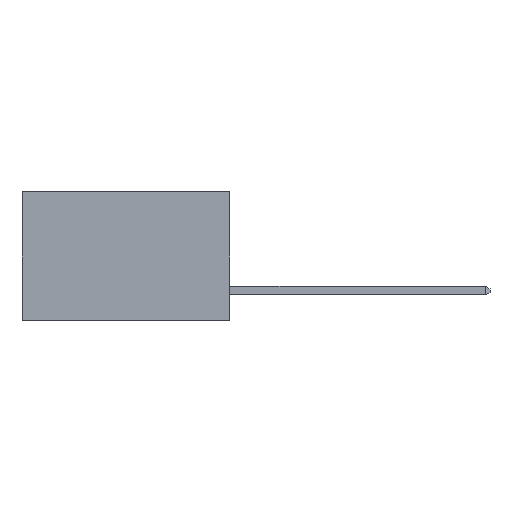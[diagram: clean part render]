
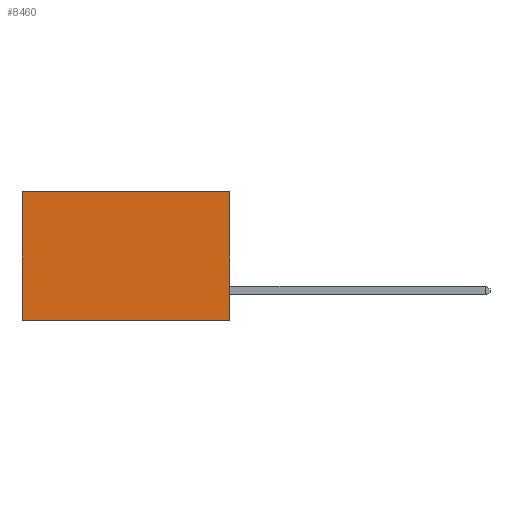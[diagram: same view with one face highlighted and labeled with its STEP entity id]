
A CAD part, left-side view. The second image highlights one B-rep face of the part: STEP entity #8460.
In plain terms, the highlighted planar face has unit normal (-1, 0, 0).
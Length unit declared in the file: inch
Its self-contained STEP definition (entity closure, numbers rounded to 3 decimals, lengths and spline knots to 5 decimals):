
#260 = VECTOR ( 'NONE', #10000, 39.37008 ) ;
#719 = VERTEX_POINT ( 'NONE', #7759 ) ;
#1228 = VERTEX_POINT ( 'NONE', #2418 ) ;
#1392 = CARTESIAN_POINT ( 'NONE',  ( 0.2615, 0., -0.37 ) ) ;
#1958 = LINE ( 'NONE', #9215, #3961 ) ;
#2029 = EDGE_CURVE ( 'NONE', #719, #5924, #1958, .T. ) ;
#2131 = CARTESIAN_POINT ( 'NONE',  ( 0.2615, 0.6, -0.37 ) ) ;
#2418 = CARTESIAN_POINT ( 'NONE',  ( 0.2615, 0., 0. ) ) ;
#2760 = ORIENTED_EDGE ( 'NONE', *, *, #7738, .F. ) ;
#2821 = ORIENTED_EDGE ( 'NONE', *, *, #2029, .T. ) ;
#2925 = LINE ( 'NONE', #7201, #260 ) ;
#3129 = EDGE_LOOP ( 'NONE', ( #2821, #2760, #8044, #6888 ) ) ;
#3337 = VECTOR ( 'NONE', #6985, 39.37008 ) ;
#3961 = VECTOR ( 'NONE', #4972, 39.37008 ) ;
#4071 = FACE_OUTER_BOUND ( 'NONE', #3129, .T. ) ;
#4377 = CARTESIAN_POINT ( 'NONE',  ( 0.2615, 0., 0. ) ) ;
#4391 = EDGE_CURVE ( 'NONE', #1228, #719, #5987, .T. ) ;
#4483 = DIRECTION ( 'NONE',  ( 0., 0., -1. ) ) ;
#4559 = DIRECTION ( 'NONE',  ( 1., 0., 0. ) ) ;
#4590 = CARTESIAN_POINT ( 'NONE',  ( 0.2615, 0., -0.37 ) ) ;
#4972 = DIRECTION ( 'NONE',  ( 0., 0., -1. ) ) ;
#5018 = PLANE ( 'NONE',  #6710 ) ;
#5579 = DIRECTION ( 'NONE',  ( 0., 1., 0. ) ) ;
#5621 = CARTESIAN_POINT ( 'NONE',  ( 0.2615, 0., -0.37 ) ) ;
#5924 = VERTEX_POINT ( 'NONE', #2131 ) ;
#5987 = LINE ( 'NONE', #4377, #7589 ) ;
#6710 = AXIS2_PLACEMENT_3D ( 'NONE', #4590, #4559, #4483 ) ;
#6888 = ORIENTED_EDGE ( 'NONE', *, *, #4391, .T. ) ;
#6985 = DIRECTION ( 'NONE',  ( 0., 0., -1. ) ) ;
#7101 = EDGE_CURVE ( 'NONE', #1228, #7464, #7654, .T. ) ;
#7201 = CARTESIAN_POINT ( 'NONE',  ( 0.2615, 0., -0.37 ) ) ;
#7464 = VERTEX_POINT ( 'NONE', #1392 ) ;
#7589 = VECTOR ( 'NONE', #5579, 39.37008 ) ;
#7654 = LINE ( 'NONE', #5621, #3337 ) ;
#7738 = EDGE_CURVE ( 'NONE', #7464, #5924, #2925, .T. ) ;
#7759 = CARTESIAN_POINT ( 'NONE',  ( 0.2615, 0.6, 0. ) ) ;
#8044 = ORIENTED_EDGE ( 'NONE', *, *, #7101, .F. ) ;
#8460 = ADVANCED_FACE ( 'NONE', ( #4071 ), #5018, .F. ) ;
#9215 = CARTESIAN_POINT ( 'NONE',  ( 0.2615, 0.6, -0.37 ) ) ;
#10000 = DIRECTION ( 'NONE',  ( 0., 1., 0. ) ) ;
